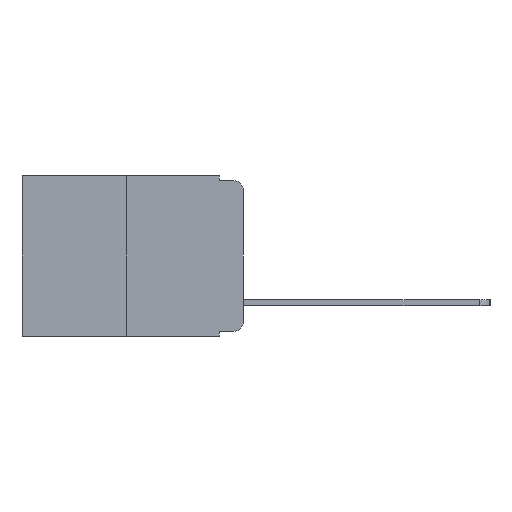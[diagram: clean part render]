
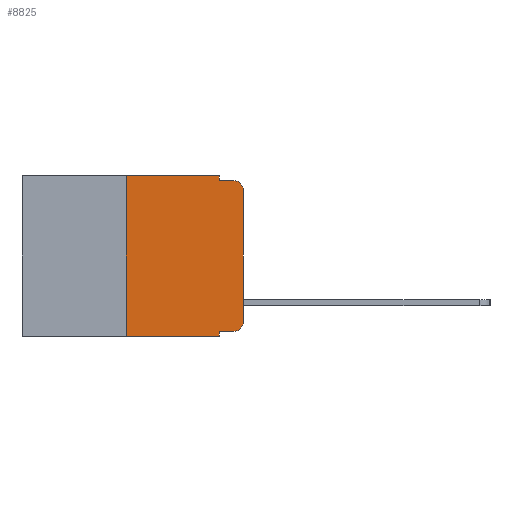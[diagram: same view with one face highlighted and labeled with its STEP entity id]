
A CAD part, left-side view. The second image highlights one B-rep face of the part: STEP entity #8825.
In plain terms, the highlighted planar face has unit normal (-1, 0, 0).
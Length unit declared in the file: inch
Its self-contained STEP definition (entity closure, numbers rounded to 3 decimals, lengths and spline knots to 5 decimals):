
#226 = DIRECTION ( 'NONE',  ( 0., -1., 0. ) ) ;
#426 = VERTEX_POINT ( 'NONE', #14382 ) ;
#612 = CARTESIAN_POINT ( 'NONE',  ( 0., 0.25, -0.343 ) ) ;
#1166 = DIRECTION ( 'NONE',  ( 0., 0., -1. ) ) ;
#1309 = EDGE_CURVE ( 'NONE', #4794, #5696, #9401, .T. ) ;
#1505 = VECTOR ( 'NONE', #1166, 39.37008 ) ;
#1669 = ORIENTED_EDGE ( 'NONE', *, *, #1964, .F. ) ;
#1744 = CARTESIAN_POINT ( 'NONE',  ( 0., 0.473, -0.343 ) ) ;
#1754 = DIRECTION ( 'NONE',  ( 0., -1., 0. ) ) ;
#1761 = CARTESIAN_POINT ( 'NONE',  ( 0., 0.02, -0.313 ) ) ;
#1964 = EDGE_CURVE ( 'NONE', #18081, #4794, #6543, .T. ) ;
#2054 = CARTESIAN_POINT ( 'NONE',  ( 0., 0.473, 0. ) ) ;
#2870 = FACE_OUTER_BOUND ( 'NONE', #7418, .T. ) ;
#3125 = CARTESIAN_POINT ( 'NONE',  ( 0., 0.051, -0.343 ) ) ;
#3218 = DIRECTION ( 'NONE',  ( 0., 0., -1. ) ) ;
#3453 = DIRECTION ( 'NONE',  ( 0., 0., -1. ) ) ;
#3516 = DIRECTION ( 'NONE',  ( 1., 0., 0. ) ) ;
#3888 = VERTEX_POINT ( 'NONE', #3125 ) ;
#3921 = CARTESIAN_POINT ( 'NONE',  ( 0., 0.051, -0.01 ) ) ;
#4003 = VERTEX_POINT ( 'NONE', #8963 ) ;
#4240 = VECTOR ( 'NONE', #10574, 39.37008 ) ;
#4794 = VERTEX_POINT ( 'NONE', #16541 ) ;
#4928 = DIRECTION ( 'NONE',  ( -1., 0., 0. ) ) ;
#4949 = EDGE_CURVE ( 'NONE', #426, #9369, #9290, .T. ) ;
#5119 = LINE ( 'NONE', #8731, #8692 ) ;
#5542 = CARTESIAN_POINT ( 'NONE',  ( 0., 0., -0.03 ) ) ;
#5696 = VERTEX_POINT ( 'NONE', #3921 ) ;
#6083 = VERTEX_POINT ( 'NONE', #7088 ) ;
#6543 = LINE ( 'NONE', #9754, #10041 ) ;
#6847 = VECTOR ( 'NONE', #11156, 39.37008 ) ;
#7088 = CARTESIAN_POINT ( 'NONE',  ( 0., 0.02, -0.01 ) ) ;
#7418 = EDGE_LOOP ( 'NONE', ( #17566, #13322, #17126, #12888, #1669, #8642, #12441, #11997, #15772, #11544 ) ) ;
#7734 = LINE ( 'NONE', #17907, #8197 ) ;
#7744 = CIRCLE ( 'NONE', #18083, 0.02 ) ;
#8197 = VECTOR ( 'NONE', #3453, 39.37008 ) ;
#8314 = EDGE_CURVE ( 'NONE', #4003, #9644, #14523, .T. ) ;
#8642 = ORIENTED_EDGE ( 'NONE', *, *, #16664, .F. ) ;
#8683 = EDGE_CURVE ( 'NONE', #17697, #3888, #15860, .T. ) ;
#8692 = VECTOR ( 'NONE', #10168, 39.37008 ) ;
#8731 = CARTESIAN_POINT ( 'NONE',  ( 0., 0.25, 0. ) ) ;
#8825 = ADVANCED_FACE ( 'NONE', ( #2870 ), #15115, .F. ) ;
#8947 = AXIS2_PLACEMENT_3D ( 'NONE', #13687, #4928, #15143 ) ;
#8963 = CARTESIAN_POINT ( 'NONE',  ( 0., 0., -0.313 ) ) ;
#9290 = LINE ( 'NONE', #16916, #16856 ) ;
#9369 = VERTEX_POINT ( 'NONE', #10551 ) ;
#9401 = LINE ( 'NONE', #9568, #1505 ) ;
#9568 = CARTESIAN_POINT ( 'NONE',  ( 0., 0.051, 0. ) ) ;
#9644 = VERTEX_POINT ( 'NONE', #5542 ) ;
#9754 = CARTESIAN_POINT ( 'NONE',  ( 0., 0.473, 0. ) ) ;
#9979 = EDGE_CURVE ( 'NONE', #9369, #4003, #7744, .T. ) ;
#10041 = VECTOR ( 'NONE', #1754, 39.37008 ) ;
#10168 = DIRECTION ( 'NONE',  ( 0., 0., 1. ) ) ;
#10551 = CARTESIAN_POINT ( 'NONE',  ( 0., 0.02, -0.333 ) ) ;
#10574 = DIRECTION ( 'NONE',  ( 0., -1., 0. ) ) ;
#10752 = CARTESIAN_POINT ( 'NONE',  ( 0., 0.25, 0. ) ) ;
#11156 = DIRECTION ( 'NONE',  ( 0., 0., 1. ) ) ;
#11544 = ORIENTED_EDGE ( 'NONE', *, *, #9979, .T. ) ;
#11914 = EDGE_CURVE ( 'NONE', #9644, #6083, #13044, .T. ) ;
#11997 = ORIENTED_EDGE ( 'NONE', *, *, #17613, .F. ) ;
#12033 = DIRECTION ( 'NONE',  ( -1., 0., 0. ) ) ;
#12441 = ORIENTED_EDGE ( 'NONE', *, *, #8683, .T. ) ;
#12575 = CARTESIAN_POINT ( 'NONE',  ( 0., 0., 0. ) ) ;
#12888 = ORIENTED_EDGE ( 'NONE', *, *, #1309, .F. ) ;
#13044 = CIRCLE ( 'NONE', #8947, 0.02 ) ;
#13322 = ORIENTED_EDGE ( 'NONE', *, *, #11914, .T. ) ;
#13687 = CARTESIAN_POINT ( 'NONE',  ( 0., 0.02, -0.03 ) ) ;
#13725 = DIRECTION ( 'NONE',  ( 0., 0., -1. ) ) ;
#13794 = EDGE_CURVE ( 'NONE', #5696, #6083, #18286, .T. ) ;
#14382 = CARTESIAN_POINT ( 'NONE',  ( 0., 0.051, -0.333 ) ) ;
#14523 = LINE ( 'NONE', #12575, #6847 ) ;
#15115 = PLANE ( 'NONE',  #18281 ) ;
#15143 = DIRECTION ( 'NONE',  ( 0., 0., -1. ) ) ;
#15772 = ORIENTED_EDGE ( 'NONE', *, *, #4949, .T. ) ;
#15860 = LINE ( 'NONE', #1744, #4240 ) ;
#16404 = CARTESIAN_POINT ( 'NONE',  ( 0., 0.051, -0.01 ) ) ;
#16541 = CARTESIAN_POINT ( 'NONE',  ( 0., 0.051, 0. ) ) ;
#16664 = EDGE_CURVE ( 'NONE', #17697, #18081, #5119, .T. ) ;
#16849 = DIRECTION ( 'NONE',  ( 0., -1., 0. ) ) ;
#16856 = VECTOR ( 'NONE', #16849, 39.37008 ) ;
#16916 = CARTESIAN_POINT ( 'NONE',  ( 0., 0.051, -0.333 ) ) ;
#17126 = ORIENTED_EDGE ( 'NONE', *, *, #13794, .F. ) ;
#17566 = ORIENTED_EDGE ( 'NONE', *, *, #8314, .T. ) ;
#17613 = EDGE_CURVE ( 'NONE', #426, #3888, #7734, .T. ) ;
#17697 = VERTEX_POINT ( 'NONE', #612 ) ;
#17870 = VECTOR ( 'NONE', #226, 39.37008 ) ;
#17907 = CARTESIAN_POINT ( 'NONE',  ( 0., 0.051, 0. ) ) ;
#18081 = VERTEX_POINT ( 'NONE', #10752 ) ;
#18083 = AXIS2_PLACEMENT_3D ( 'NONE', #1761, #12033, #3218 ) ;
#18281 = AXIS2_PLACEMENT_3D ( 'NONE', #2054, #3516, #13725 ) ;
#18286 = LINE ( 'NONE', #16404, #17870 ) ;
